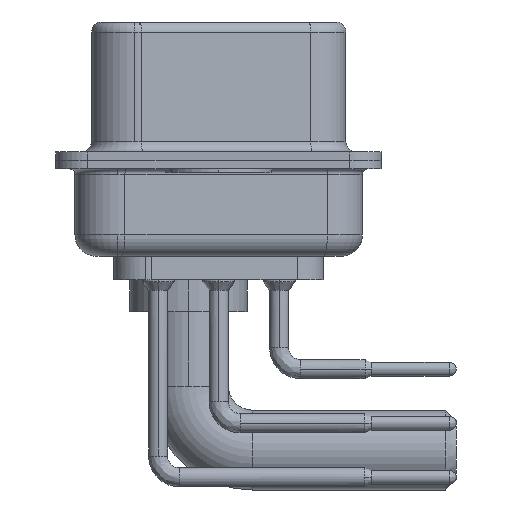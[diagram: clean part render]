
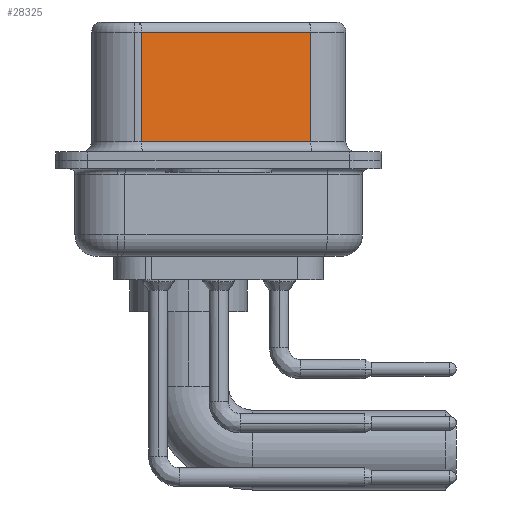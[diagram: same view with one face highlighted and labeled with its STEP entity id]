
A CAD part, left-side view. The second image highlights one B-rep face of the part: STEP entity #28325.
In plain terms, the highlighted planar face has unit normal (-0.985, -0.174, 0).
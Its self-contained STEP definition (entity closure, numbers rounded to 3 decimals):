
#1721 = VECTOR ( 'NONE', #4034, 1000. ) ;
#3340 = ORIENTED_EDGE ( 'NONE', *, *, #7050, .F. ) ;
#4034 = DIRECTION ( 'NONE',  ( 0.174, -0.985, 0. ) ) ;
#5491 = LINE ( 'NONE', #28851, #20743 ) ;
#6200 = DIRECTION ( 'NONE',  ( 0.985, 0.174, 0. ) ) ;
#6217 = VERTEX_POINT ( 'NONE', #31441 ) ;
#7050 = EDGE_CURVE ( 'NONE', #9451, #28175, #21025, .T. ) ;
#8360 = VECTOR ( 'NONE', #26430, 1000. ) ;
#9451 = VERTEX_POINT ( 'NONE', #28229 ) ;
#9489 = EDGE_CURVE ( 'NONE', #20132, #28175, #27559, .T. ) ;
#13665 = DIRECTION ( 'NONE',  ( 0., 0., -1. ) ) ;
#13907 = ORIENTED_EDGE ( 'NONE', *, *, #27020, .T. ) ;
#14485 = CARTESIAN_POINT ( 'NONE',  ( 5.132, -4.322, 0.9 ) ) ;
#15160 = CARTESIAN_POINT ( 'NONE',  ( 5.132, -4.322, 6.52 ) ) ;
#15766 = AXIS2_PLACEMENT_3D ( 'NONE', #15160, #6200, #21874 ) ;
#15829 = CARTESIAN_POINT ( 'NONE',  ( 5.132, -4.322, 6.52 ) ) ;
#16288 = LINE ( 'NONE', #19063, #21562 ) ;
#17581 = ORIENTED_EDGE ( 'NONE', *, *, #33749, .T. ) ;
#18516 = ORIENTED_EDGE ( 'NONE', *, *, #9489, .T. ) ;
#18924 = FACE_OUTER_BOUND ( 'NONE', #30832, .T. ) ;
#19063 = CARTESIAN_POINT ( 'NONE',  ( 3.73, 3.628, 6.52 ) ) ;
#20132 = VERTEX_POINT ( 'NONE', #32116 ) ;
#20743 = VECTOR ( 'NONE', #31812, 1000. ) ;
#21025 = LINE ( 'NONE', #15829, #8360 ) ;
#21562 = VECTOR ( 'NONE', #13665, 1000. ) ;
#21874 = DIRECTION ( 'NONE',  ( -0.174, 0.985, 0. ) ) ;
#26430 = DIRECTION ( 'NONE',  ( 0., 0., -1. ) ) ;
#27020 = EDGE_CURVE ( 'NONE', #9451, #6217, #5491, .T. ) ;
#27559 = LINE ( 'NONE', #27911, #1721 ) ;
#27911 = CARTESIAN_POINT ( 'NONE',  ( 5.132, -4.322, 0.9 ) ) ;
#28175 = VERTEX_POINT ( 'NONE', #14485 ) ;
#28229 = CARTESIAN_POINT ( 'NONE',  ( 5.132, -4.322, 6.02 ) ) ;
#28325 = ADVANCED_FACE ( 'NONE', ( #18924 ), #31511, .F. ) ;
#28851 = CARTESIAN_POINT ( 'NONE',  ( 5.132, -4.322, 6.02 ) ) ;
#30832 = EDGE_LOOP ( 'NONE', ( #3340, #13907, #17581, #18516 ) ) ;
#31441 = CARTESIAN_POINT ( 'NONE',  ( 3.73, 3.628, 6.02 ) ) ;
#31511 = PLANE ( 'NONE',  #15766 ) ;
#31812 = DIRECTION ( 'NONE',  ( -0.174, 0.985, 0. ) ) ;
#32116 = CARTESIAN_POINT ( 'NONE',  ( 3.73, 3.628, 0.9 ) ) ;
#33749 = EDGE_CURVE ( 'NONE', #6217, #20132, #16288, .T. ) ;
